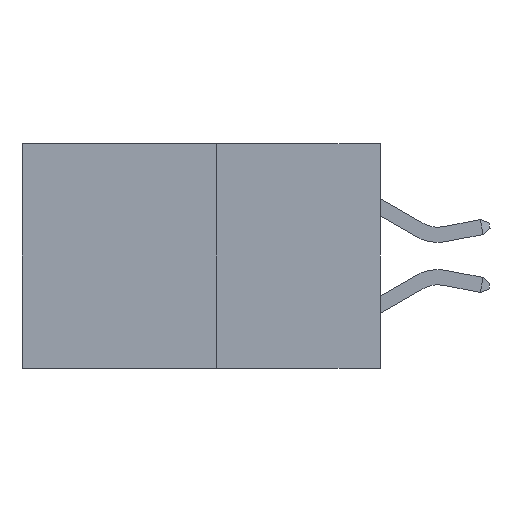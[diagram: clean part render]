
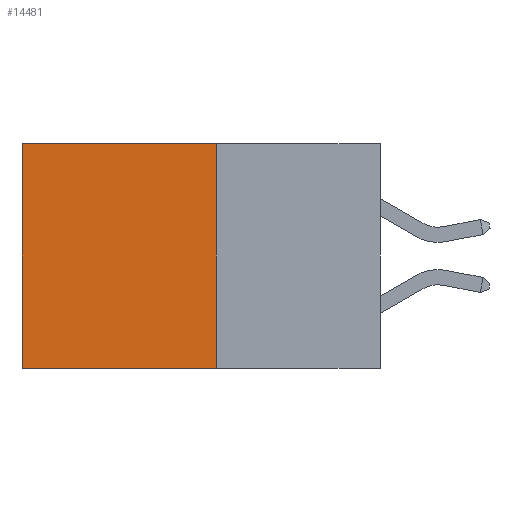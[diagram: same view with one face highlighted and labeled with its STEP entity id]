
A CAD part, left-side view. The second image highlights one B-rep face of the part: STEP entity #14481.
In plain terms, the highlighted planar face has unit normal (-1, 0, 0).
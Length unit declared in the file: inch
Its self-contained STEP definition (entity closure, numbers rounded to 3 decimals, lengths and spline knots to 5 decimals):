
#619 = DIRECTION ( 'NONE',  ( 1., 0., 0. ) ) ;
#911 = VECTOR ( 'NONE', #5132, 39.37008 ) ;
#1804 = CARTESIAN_POINT ( 'NONE',  ( 0.277, 0.27, -0.37 ) ) ;
#1913 = EDGE_CURVE ( 'NONE', #7465, #19261, #19516, .T. ) ;
#2097 = DIRECTION ( 'NONE',  ( 0., 0., -1. ) ) ;
#2734 = VECTOR ( 'NONE', #5474, 39.37008 ) ;
#3243 = LINE ( 'NONE', #3854, #2734 ) ;
#3854 = CARTESIAN_POINT ( 'NONE',  ( 0.277, 0.27, 0. ) ) ;
#5132 = DIRECTION ( 'NONE',  ( 0., 1., 0. ) ) ;
#5287 = LINE ( 'NONE', #1804, #911 ) ;
#5325 = EDGE_CURVE ( 'NONE', #6021, #19261, #5287, .T. ) ;
#5474 = DIRECTION ( 'NONE',  ( 0., 1., 0. ) ) ;
#5506 = EDGE_CURVE ( 'NONE', #16716, #7465, #3243, .T. ) ;
#5848 = AXIS2_PLACEMENT_3D ( 'NONE', #8518, #619, #11620 ) ;
#6021 = VERTEX_POINT ( 'NONE', #8120 ) ;
#6195 = CARTESIAN_POINT ( 'NONE',  ( 0.277, 0.59, -0.37 ) ) ;
#7419 = CARTESIAN_POINT ( 'NONE',  ( 0.277, 0.59, -0.37 ) ) ;
#7465 = VERTEX_POINT ( 'NONE', #9079 ) ;
#8120 = CARTESIAN_POINT ( 'NONE',  ( 0.277, 0.27, -0.37 ) ) ;
#8518 = CARTESIAN_POINT ( 'NONE',  ( 0.277, 0.27, -0.37 ) ) ;
#9079 = CARTESIAN_POINT ( 'NONE',  ( 0.277, 0.59, 0. ) ) ;
#9802 = ORIENTED_EDGE ( 'NONE', *, *, #5506, .T. ) ;
#9819 = DIRECTION ( 'NONE',  ( 0., 0., -1. ) ) ;
#10098 = PLANE ( 'NONE',  #5848 ) ;
#10911 = VECTOR ( 'NONE', #2097, 39.37008 ) ;
#11366 = VECTOR ( 'NONE', #9819, 39.37008 ) ;
#11620 = DIRECTION ( 'NONE',  ( 0., 0., -1. ) ) ;
#12452 = CARTESIAN_POINT ( 'NONE',  ( 0.277, 0.27, 0. ) ) ;
#14123 = EDGE_LOOP ( 'NONE', ( #19853, #15596, #16715, #9802 ) ) ;
#14481 = ADVANCED_FACE ( 'NONE', ( #19042 ), #10098, .F. ) ;
#14911 = EDGE_CURVE ( 'NONE', #16716, #6021, #19019, .T. ) ;
#15596 = ORIENTED_EDGE ( 'NONE', *, *, #5325, .F. ) ;
#16715 = ORIENTED_EDGE ( 'NONE', *, *, #14911, .F. ) ;
#16716 = VERTEX_POINT ( 'NONE', #12452 ) ;
#18947 = CARTESIAN_POINT ( 'NONE',  ( 0.277, 0.27, -0.37 ) ) ;
#19019 = LINE ( 'NONE', #18947, #11366 ) ;
#19042 = FACE_OUTER_BOUND ( 'NONE', #14123, .T. ) ;
#19261 = VERTEX_POINT ( 'NONE', #6195 ) ;
#19516 = LINE ( 'NONE', #7419, #10911 ) ;
#19853 = ORIENTED_EDGE ( 'NONE', *, *, #1913, .T. ) ;
